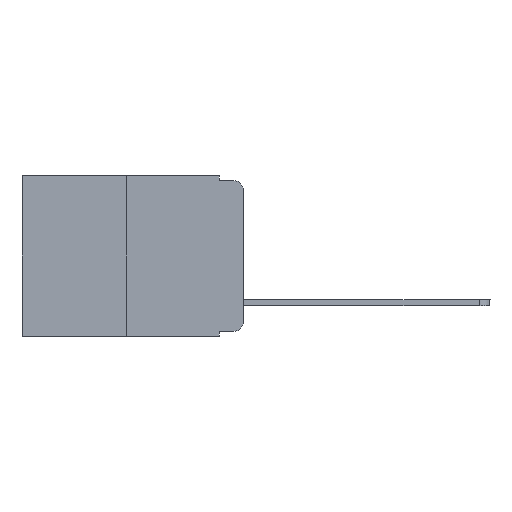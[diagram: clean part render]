
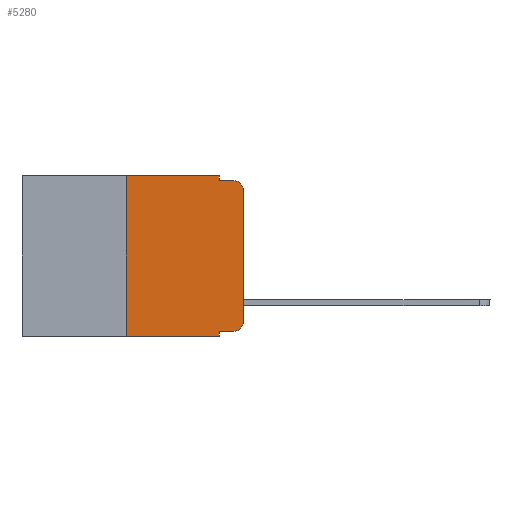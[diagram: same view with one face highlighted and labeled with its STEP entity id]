
A CAD part, left-side view. The second image highlights one B-rep face of the part: STEP entity #5280.
In plain terms, the highlighted planar face has unit normal (-1, 0, 0).
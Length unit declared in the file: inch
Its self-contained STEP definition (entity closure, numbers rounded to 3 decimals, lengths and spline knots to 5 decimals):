
#62 = CARTESIAN_POINT ( 'NONE',  ( 0., 0., 0. ) ) ;
#207 = VECTOR ( 'NONE', #9382, 39.37008 ) ;
#347 = EDGE_CURVE ( 'NONE', #5467, #6887, #8515, .T. ) ;
#467 = ORIENTED_EDGE ( 'NONE', *, *, #347, .F. ) ;
#893 = ORIENTED_EDGE ( 'NONE', *, *, #4032, .F. ) ;
#965 = DIRECTION ( 'NONE',  ( 0., -1., 0. ) ) ;
#1030 = ORIENTED_EDGE ( 'NONE', *, *, #8308, .F. ) ;
#1123 = DIRECTION ( 'NONE',  ( -1., 0., 0. ) ) ;
#1134 = DIRECTION ( 'NONE',  ( 0., -1., 0. ) ) ;
#1239 = CARTESIAN_POINT ( 'NONE',  ( 0., 0.25, 0. ) ) ;
#1445 = VECTOR ( 'NONE', #6143, 39.37008 ) ;
#1655 = ORIENTED_EDGE ( 'NONE', *, *, #11649, .T. ) ;
#1671 = CIRCLE ( 'NONE', #9220, 0.02 ) ;
#1674 = CARTESIAN_POINT ( 'NONE',  ( 0., 0.051, -0.01 ) ) ;
#1731 = VERTEX_POINT ( 'NONE', #6100 ) ;
#1817 = DIRECTION ( 'NONE',  ( 0., 0., -1. ) ) ;
#2132 = CARTESIAN_POINT ( 'NONE',  ( 0., 0.051, 0. ) ) ;
#2338 = PLANE ( 'NONE',  #4945 ) ;
#2429 = VERTEX_POINT ( 'NONE', #2662 ) ;
#2533 = VERTEX_POINT ( 'NONE', #5630 ) ;
#2585 = EDGE_CURVE ( 'NONE', #6456, #12001, #12020, .T. ) ;
#2605 = EDGE_CURVE ( 'NONE', #11695, #2429, #5216, .T. ) ;
#2662 = CARTESIAN_POINT ( 'NONE',  ( 0., 0., -0.03 ) ) ;
#3275 = ORIENTED_EDGE ( 'NONE', *, *, #5754, .T. ) ;
#3313 = DIRECTION ( 'NONE',  ( 0., -1., 0. ) ) ;
#3376 = CARTESIAN_POINT ( 'NONE',  ( 0., 0.051, -0.333 ) ) ;
#3407 = VECTOR ( 'NONE', #10972, 39.37008 ) ;
#3463 = AXIS2_PLACEMENT_3D ( 'NONE', #6746, #1123, #8679 ) ;
#3657 = VECTOR ( 'NONE', #5142, 39.37008 ) ;
#3992 = ORIENTED_EDGE ( 'NONE', *, *, #5740, .F. ) ;
#4032 = EDGE_CURVE ( 'NONE', #4900, #8677, #5862, .T. ) ;
#4075 = CIRCLE ( 'NONE', #3463, 0.02 ) ;
#4163 = ORIENTED_EDGE ( 'NONE', *, *, #7313, .T. ) ;
#4597 = CARTESIAN_POINT ( 'NONE',  ( 0., 0.02, -0.313 ) ) ;
#4641 = VECTOR ( 'NONE', #3313, 39.37008 ) ;
#4869 = CARTESIAN_POINT ( 'NONE',  ( 0., 0.473, 0. ) ) ;
#4900 = VERTEX_POINT ( 'NONE', #1674 ) ;
#4945 = AXIS2_PLACEMENT_3D ( 'NONE', #10643, #7044, #10729 ) ;
#5138 = EDGE_CURVE ( 'NONE', #6887, #2533, #8647, .T. ) ;
#5142 = DIRECTION ( 'NONE',  ( 0., 0., 1. ) ) ;
#5216 = LINE ( 'NONE', #62, #207 ) ;
#5280 = ADVANCED_FACE ( 'NONE', ( #5407 ), #2338, .F. ) ;
#5407 = FACE_OUTER_BOUND ( 'NONE', #9237, .T. ) ;
#5442 = CARTESIAN_POINT ( 'NONE',  ( 0., 0.25, -0.343 ) ) ;
#5467 = VERTEX_POINT ( 'NONE', #5442 ) ;
#5630 = CARTESIAN_POINT ( 'NONE',  ( 0., 0.051, 0. ) ) ;
#5740 = EDGE_CURVE ( 'NONE', #6456, #1731, #11295, .T. ) ;
#5754 = EDGE_CURVE ( 'NONE', #2429, #8677, #4075, .T. ) ;
#5862 = LINE ( 'NONE', #10854, #1445 ) ;
#5946 = ORIENTED_EDGE ( 'NONE', *, *, #2605, .T. ) ;
#6100 = CARTESIAN_POINT ( 'NONE',  ( 0., 0.051, -0.343 ) ) ;
#6143 = DIRECTION ( 'NONE',  ( 0., -1., 0. ) ) ;
#6260 = CARTESIAN_POINT ( 'NONE',  ( 0., 0.473, -0.343 ) ) ;
#6348 = ORIENTED_EDGE ( 'NONE', *, *, #5138, .F. ) ;
#6456 = VERTEX_POINT ( 'NONE', #3376 ) ;
#6625 = CARTESIAN_POINT ( 'NONE',  ( 0., 0.02, -0.01 ) ) ;
#6746 = CARTESIAN_POINT ( 'NONE',  ( 0., 0.02, -0.03 ) ) ;
#6887 = VERTEX_POINT ( 'NONE', #1239 ) ;
#7044 = DIRECTION ( 'NONE',  ( 1., 0., 0. ) ) ;
#7313 = EDGE_CURVE ( 'NONE', #12001, #11695, #1671, .T. ) ;
#7433 = DIRECTION ( 'NONE',  ( -1., 0., 0. ) ) ;
#7442 = VECTOR ( 'NONE', #7728, 39.37008 ) ;
#7512 = CARTESIAN_POINT ( 'NONE',  ( 0., 0.02, -0.333 ) ) ;
#7728 = DIRECTION ( 'NONE',  ( 0., 0., -1. ) ) ;
#7980 = CARTESIAN_POINT ( 'NONE',  ( 0., 0., -0.313 ) ) ;
#8308 = EDGE_CURVE ( 'NONE', #2533, #4900, #10622, .T. ) ;
#8309 = VECTOR ( 'NONE', #965, 39.37008 ) ;
#8478 = LINE ( 'NONE', #6260, #4641 ) ;
#8515 = LINE ( 'NONE', #10556, #3657 ) ;
#8647 = LINE ( 'NONE', #4869, #9401 ) ;
#8677 = VERTEX_POINT ( 'NONE', #6625 ) ;
#8679 = DIRECTION ( 'NONE',  ( 0., 0., -1. ) ) ;
#9086 = ORIENTED_EDGE ( 'NONE', *, *, #2585, .T. ) ;
#9198 = CARTESIAN_POINT ( 'NONE',  ( 0., 0.051, 0. ) ) ;
#9220 = AXIS2_PLACEMENT_3D ( 'NONE', #4597, #7433, #1817 ) ;
#9237 = EDGE_LOOP ( 'NONE', ( #5946, #3275, #893, #1030, #6348, #467, #1655, #3992, #9086, #4163 ) ) ;
#9382 = DIRECTION ( 'NONE',  ( 0., 0., 1. ) ) ;
#9401 = VECTOR ( 'NONE', #1134, 39.37008 ) ;
#10556 = CARTESIAN_POINT ( 'NONE',  ( 0., 0.25, 0. ) ) ;
#10622 = LINE ( 'NONE', #9198, #3407 ) ;
#10643 = CARTESIAN_POINT ( 'NONE',  ( 0., 0.473, 0. ) ) ;
#10729 = DIRECTION ( 'NONE',  ( 0., 0., -1. ) ) ;
#10854 = CARTESIAN_POINT ( 'NONE',  ( 0., 0.051, -0.01 ) ) ;
#10972 = DIRECTION ( 'NONE',  ( 0., 0., -1. ) ) ;
#11295 = LINE ( 'NONE', #2132, #7442 ) ;
#11357 = CARTESIAN_POINT ( 'NONE',  ( 0., 0.051, -0.333 ) ) ;
#11649 = EDGE_CURVE ( 'NONE', #5467, #1731, #8478, .T. ) ;
#11695 = VERTEX_POINT ( 'NONE', #7980 ) ;
#12001 = VERTEX_POINT ( 'NONE', #7512 ) ;
#12020 = LINE ( 'NONE', #11357, #8309 ) ;
